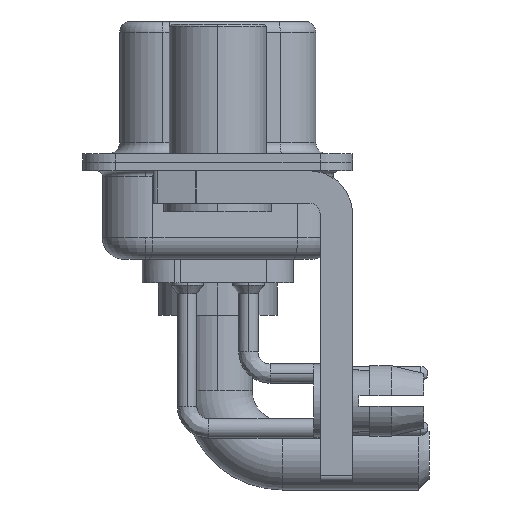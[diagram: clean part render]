
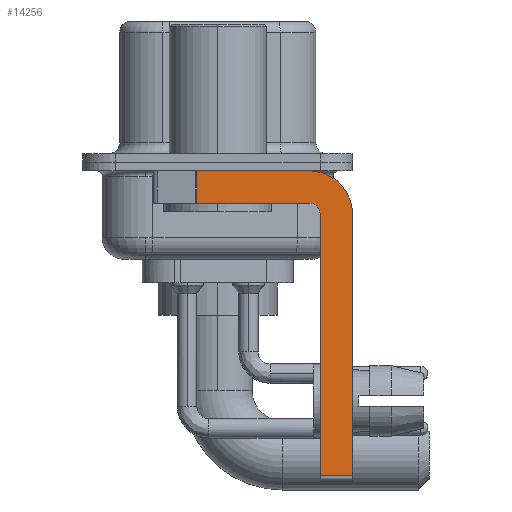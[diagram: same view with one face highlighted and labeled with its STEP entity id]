
A CAD part, left-side view. The second image highlights one B-rep face of the part: STEP entity #14256.
In plain terms, the highlighted planar face has unit normal (-1, 0, 0).
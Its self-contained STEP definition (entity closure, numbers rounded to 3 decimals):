
#65 = CARTESIAN_POINT ( 'NONE',  ( -2.9, -4.25, -1.9 ) ) ;
#395 = LINE ( 'NONE', #7631, #15571 ) ;
#1435 = CARTESIAN_POINT ( 'NONE',  ( -2.9, -4.25, -2.4 ) ) ;
#1806 = AXIS2_PLACEMENT_3D ( 'NONE', #13686, #19019, #20929 ) ;
#1851 = VERTEX_POINT ( 'NONE', #6607 ) ;
#2033 = EDGE_CURVE ( 'NONE', #22150, #22007, #8035, .T. ) ;
#2660 = VERTEX_POINT ( 'NONE', #19516 ) ;
#2907 = ORIENTED_EDGE ( 'NONE', *, *, #13752, .F. ) ;
#2921 = VERTEX_POINT ( 'NONE', #18091 ) ;
#2986 = DIRECTION ( 'NONE',  ( 0., 0., -1. ) ) ;
#3844 = LINE ( 'NONE', #65, #14024 ) ;
#3861 = ORIENTED_EDGE ( 'NONE', *, *, #2033, .F. ) ;
#4176 = VERTEX_POINT ( 'NONE', #11192 ) ;
#4561 = VECTOR ( 'NONE', #17604, 1000. ) ;
#5174 = VERTEX_POINT ( 'NONE', #21571 ) ;
#5946 = CARTESIAN_POINT ( 'NONE',  ( -2.9, -4.75, -14.55 ) ) ;
#6036 = EDGE_CURVE ( 'NONE', #2660, #13668, #16816, .T. ) ;
#6171 = CARTESIAN_POINT ( 'NONE',  ( -2.9, -4.25, -2.4 ) ) ;
#6204 = DIRECTION ( 'NONE',  ( 0., 0., -1. ) ) ;
#6290 = LINE ( 'NONE', #22316, #15695 ) ;
#6607 = CARTESIAN_POINT ( 'NONE',  ( -2.9, -4.25, -1.9 ) ) ;
#6740 = CIRCLE ( 'NONE', #1806, 0.5 ) ;
#7514 = CARTESIAN_POINT ( 'NONE',  ( -2.9, 0.978, -1.9 ) ) ;
#7631 = CARTESIAN_POINT ( 'NONE',  ( -2.9, -6.25, -2.4 ) ) ;
#8035 = LINE ( 'NONE', #11479, #22522 ) ;
#8352 = ORIENTED_EDGE ( 'NONE', *, *, #21552, .F. ) ;
#8773 = VECTOR ( 'NONE', #11330, 1000. ) ;
#8912 = LINE ( 'NONE', #21060, #4561 ) ;
#10564 = DIRECTION ( 'NONE',  ( 1., 0., 0. ) ) ;
#11192 = CARTESIAN_POINT ( 'NONE',  ( -2.9, -6.25, -2.4 ) ) ;
#11330 = DIRECTION ( 'NONE',  ( 0., 0., -1. ) ) ;
#11479 = CARTESIAN_POINT ( 'NONE',  ( -2.9, -4.75, -14.8 ) ) ;
#11628 = DIRECTION ( 'NONE',  ( 0., -1., 0. ) ) ;
#11636 = FACE_OUTER_BOUND ( 'NONE', #18226, .T. ) ;
#11764 = AXIS2_PLACEMENT_3D ( 'NONE', #1435, #10564, #2986 ) ;
#11909 = EDGE_CURVE ( 'NONE', #22007, #1851, #6740, .T. ) ;
#12575 = ORIENTED_EDGE ( 'NONE', *, *, #6036, .T. ) ;
#13623 = DIRECTION ( 'NONE',  ( 0., 0., 1. ) ) ;
#13658 = DIRECTION ( 'NONE',  ( 0., 0., -1. ) ) ;
#13668 = VERTEX_POINT ( 'NONE', #7514 ) ;
#13686 = CARTESIAN_POINT ( 'NONE',  ( -2.9, -4.25, -2.4 ) ) ;
#13752 = EDGE_CURVE ( 'NONE', #4176, #5174, #395, .T. ) ;
#14024 = VECTOR ( 'NONE', #14312, 1000. ) ;
#14256 = ADVANCED_FACE ( 'NONE', ( #11636 ), #18884, .F. ) ;
#14312 = DIRECTION ( 'NONE',  ( 0., 1., 0. ) ) ;
#15516 = ORIENTED_EDGE ( 'NONE', *, *, #19474, .T. ) ;
#15571 = VECTOR ( 'NONE', #6204, 1000. ) ;
#15695 = VECTOR ( 'NONE', #11628, 1000. ) ;
#15942 = CIRCLE ( 'NONE', #11764, 2. ) ;
#16816 = LINE ( 'NONE', #20373, #8773 ) ;
#17236 = DIRECTION ( 'NONE',  ( 1., 0., 0. ) ) ;
#17604 = DIRECTION ( 'NONE',  ( 0., -1., 0. ) ) ;
#17963 = ORIENTED_EDGE ( 'NONE', *, *, #11909, .F. ) ;
#18091 = CARTESIAN_POINT ( 'NONE',  ( -2.9, -4.25, -0.4 ) ) ;
#18226 = EDGE_LOOP ( 'NONE', ( #21041, #12575, #8352, #17963, #3861, #15516, #2907, #20845 ) ) ;
#18456 = EDGE_CURVE ( 'NONE', #2660, #2921, #6290, .T. ) ;
#18884 = PLANE ( 'NONE',  #22421 ) ;
#19019 = DIRECTION ( 'NONE',  ( -1., 0., 0. ) ) ;
#19474 = EDGE_CURVE ( 'NONE', #22150, #5174, #8912, .T. ) ;
#19516 = CARTESIAN_POINT ( 'NONE',  ( -2.9, 0.978, -0.4 ) ) ;
#19566 = EDGE_CURVE ( 'NONE', #2921, #4176, #15942, .T. ) ;
#20373 = CARTESIAN_POINT ( 'NONE',  ( -2.9, 0.978, -1.9 ) ) ;
#20845 = ORIENTED_EDGE ( 'NONE', *, *, #19566, .F. ) ;
#20929 = DIRECTION ( 'NONE',  ( 0., 0., 1. ) ) ;
#21041 = ORIENTED_EDGE ( 'NONE', *, *, #18456, .F. ) ;
#21060 = CARTESIAN_POINT ( 'NONE',  ( -2.9, -4.25, -14.55 ) ) ;
#21552 = EDGE_CURVE ( 'NONE', #1851, #13668, #3844, .T. ) ;
#21571 = CARTESIAN_POINT ( 'NONE',  ( -2.9, -6.25, -14.55 ) ) ;
#21879 = CARTESIAN_POINT ( 'NONE',  ( -2.9, -4.75, -2.4 ) ) ;
#22007 = VERTEX_POINT ( 'NONE', #21879 ) ;
#22150 = VERTEX_POINT ( 'NONE', #5946 ) ;
#22316 = CARTESIAN_POINT ( 'NONE',  ( -2.9, 3., -0.4 ) ) ;
#22421 = AXIS2_PLACEMENT_3D ( 'NONE', #6171, #17236, #13658 ) ;
#22522 = VECTOR ( 'NONE', #13623, 1000. ) ;
